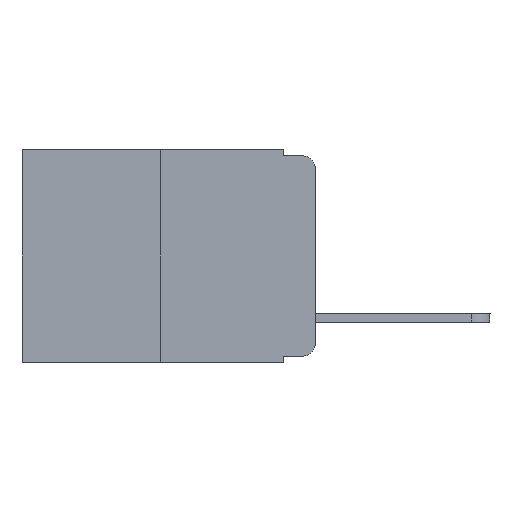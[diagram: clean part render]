
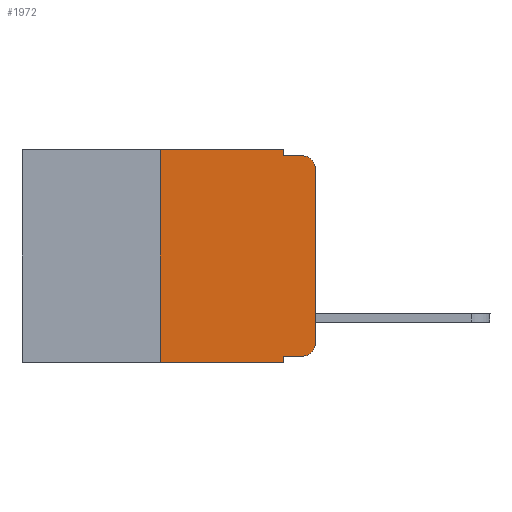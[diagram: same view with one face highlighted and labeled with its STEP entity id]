
A CAD part, left-side view. The second image highlights one B-rep face of the part: STEP entity #1972.
In plain terms, the highlighted planar face has unit normal (-1, 0, 0).
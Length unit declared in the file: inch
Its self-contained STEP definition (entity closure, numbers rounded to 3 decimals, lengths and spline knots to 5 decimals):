
#208 = DIRECTION ( 'NONE',  ( 0., 0., 1. ) ) ;
#659 = LINE ( 'NONE', #13359, #13263 ) ;
#694 = CARTESIAN_POINT ( 'NONE',  ( 0., 0.473, 0. ) ) ;
#1264 = DIRECTION ( 'NONE',  ( 0., 0., -1. ) ) ;
#1490 = CARTESIAN_POINT ( 'NONE',  ( 0., 0.051, -0.333 ) ) ;
#1658 = DIRECTION ( 'NONE',  ( 0., -1., 0. ) ) ;
#1783 = CARTESIAN_POINT ( 'NONE',  ( 0., 0.25, -0.343 ) ) ;
#1972 = ADVANCED_FACE ( 'NONE', ( #10226 ), #14744, .F. ) ;
#3472 = VERTEX_POINT ( 'NONE', #1783 ) ;
#3573 = ORIENTED_EDGE ( 'NONE', *, *, #5181, .T. ) ;
#3999 = CARTESIAN_POINT ( 'NONE',  ( 0., 0.051, -0.333 ) ) ;
#4110 = DIRECTION ( 'NONE',  ( -1., 0., 0. ) ) ;
#4302 = ORIENTED_EDGE ( 'NONE', *, *, #16141, .F. ) ;
#4472 = ORIENTED_EDGE ( 'NONE', *, *, #11755, .F. ) ;
#5054 = VERTEX_POINT ( 'NONE', #16000 ) ;
#5181 = EDGE_CURVE ( 'NONE', #12700, #6985, #9974, .T. ) ;
#5601 = DIRECTION ( 'NONE',  ( 0., 0., -1. ) ) ;
#5642 = EDGE_CURVE ( 'NONE', #3472, #6374, #10042, .T. ) ;
#5672 = CIRCLE ( 'NONE', #19744, 0.02 ) ;
#5918 = VECTOR ( 'NONE', #6756, 39.37008 ) ;
#6089 = CARTESIAN_POINT ( 'NONE',  ( 0., 0.25, 0. ) ) ;
#6374 = VERTEX_POINT ( 'NONE', #12897 ) ;
#6541 = CARTESIAN_POINT ( 'NONE',  ( 0., 0., -0.313 ) ) ;
#6551 = VECTOR ( 'NONE', #19819, 39.37008 ) ;
#6756 = DIRECTION ( 'NONE',  ( 0., -1., 0. ) ) ;
#6985 = VERTEX_POINT ( 'NONE', #12706 ) ;
#7317 = ORIENTED_EDGE ( 'NONE', *, *, #8917, .T. ) ;
#7386 = LINE ( 'NONE', #13646, #15836 ) ;
#7687 = VERTEX_POINT ( 'NONE', #7826 ) ;
#7826 = CARTESIAN_POINT ( 'NONE',  ( 0., 0.051, 0. ) ) ;
#8435 = DIRECTION ( 'NONE',  ( 0., 0., -1. ) ) ;
#8522 = ORIENTED_EDGE ( 'NONE', *, *, #5642, .T. ) ;
#8561 = DIRECTION ( 'NONE',  ( -1., 0., 0. ) ) ;
#8579 = CARTESIAN_POINT ( 'NONE',  ( 0., 0.473, -0.343 ) ) ;
#8917 = EDGE_CURVE ( 'NONE', #20241, #9786, #17738, .T. ) ;
#9378 = CARTESIAN_POINT ( 'NONE',  ( 0., 0.051, -0.01 ) ) ;
#9562 = CARTESIAN_POINT ( 'NONE',  ( 0., 0.473, 0. ) ) ;
#9786 = VERTEX_POINT ( 'NONE', #18335 ) ;
#9863 = DIRECTION ( 'NONE',  ( 0., -1., 0. ) ) ;
#9974 = LINE ( 'NONE', #3999, #16720 ) ;
#10042 = LINE ( 'NONE', #8579, #5918 ) ;
#10110 = CARTESIAN_POINT ( 'NONE',  ( 0., 0.02, -0.03 ) ) ;
#10226 = FACE_OUTER_BOUND ( 'NONE', #14265, .T. ) ;
#10424 = CARTESIAN_POINT ( 'NONE',  ( 0., 0., -0.03 ) ) ;
#11413 = CARTESIAN_POINT ( 'NONE',  ( 0., 0.051, -0.01 ) ) ;
#11673 = VERTEX_POINT ( 'NONE', #9378 ) ;
#11755 = EDGE_CURVE ( 'NONE', #12700, #6374, #659, .T. ) ;
#12264 = ORIENTED_EDGE ( 'NONE', *, *, #19534, .T. ) ;
#12394 = VECTOR ( 'NONE', #1658, 39.37008 ) ;
#12700 = VERTEX_POINT ( 'NONE', #1490 ) ;
#12706 = CARTESIAN_POINT ( 'NONE',  ( 0., 0.02, -0.333 ) ) ;
#12897 = CARTESIAN_POINT ( 'NONE',  ( 0., 0.051, -0.343 ) ) ;
#13050 = LINE ( 'NONE', #11413, #14045 ) ;
#13263 = VECTOR ( 'NONE', #8435, 39.37008 ) ;
#13359 = CARTESIAN_POINT ( 'NONE',  ( 0., 0.051, 0. ) ) ;
#13646 = CARTESIAN_POINT ( 'NONE',  ( 0., 0., 0. ) ) ;
#13983 = LINE ( 'NONE', #18255, #14373 ) ;
#14045 = VECTOR ( 'NONE', #16410, 39.37008 ) ;
#14265 = EDGE_LOOP ( 'NONE', ( #12264, #7317, #20155, #17011, #14836, #4302, #8522, #4472, #3573, #19899 ) ) ;
#14373 = VECTOR ( 'NONE', #1264, 39.37008 ) ;
#14385 = LINE ( 'NONE', #9562, #12394 ) ;
#14744 = PLANE ( 'NONE',  #20059 ) ;
#14786 = EDGE_CURVE ( 'NONE', #7687, #11673, #13983, .T. ) ;
#14836 = ORIENTED_EDGE ( 'NONE', *, *, #14855, .F. ) ;
#14839 = DIRECTION ( 'NONE',  ( 0., 0., -1. ) ) ;
#14855 = EDGE_CURVE ( 'NONE', #5054, #7687, #14385, .T. ) ;
#15091 = EDGE_CURVE ( 'NONE', #11673, #9786, #13050, .T. ) ;
#15764 = AXIS2_PLACEMENT_3D ( 'NONE', #10110, #8561, #14839 ) ;
#15836 = VECTOR ( 'NONE', #208, 39.37008 ) ;
#16000 = CARTESIAN_POINT ( 'NONE',  ( 0., 0.25, 0. ) ) ;
#16141 = EDGE_CURVE ( 'NONE', #3472, #5054, #18670, .T. ) ;
#16410 = DIRECTION ( 'NONE',  ( 0., -1., 0. ) ) ;
#16568 = DIRECTION ( 'NONE',  ( 1., 0., 0. ) ) ;
#16720 = VECTOR ( 'NONE', #9863, 39.37008 ) ;
#17011 = ORIENTED_EDGE ( 'NONE', *, *, #14786, .F. ) ;
#17036 = VERTEX_POINT ( 'NONE', #6541 ) ;
#17738 = CIRCLE ( 'NONE', #15764, 0.02 ) ;
#18139 = CARTESIAN_POINT ( 'NONE',  ( 0., 0.02, -0.313 ) ) ;
#18255 = CARTESIAN_POINT ( 'NONE',  ( 0., 0.051, 0. ) ) ;
#18335 = CARTESIAN_POINT ( 'NONE',  ( 0., 0.02, -0.01 ) ) ;
#18448 = DIRECTION ( 'NONE',  ( 0., 0., -1. ) ) ;
#18670 = LINE ( 'NONE', #6089, #6551 ) ;
#19406 = EDGE_CURVE ( 'NONE', #6985, #17036, #5672, .T. ) ;
#19534 = EDGE_CURVE ( 'NONE', #17036, #20241, #7386, .T. ) ;
#19744 = AXIS2_PLACEMENT_3D ( 'NONE', #18139, #4110, #18448 ) ;
#19819 = DIRECTION ( 'NONE',  ( 0., 0., 1. ) ) ;
#19899 = ORIENTED_EDGE ( 'NONE', *, *, #19406, .T. ) ;
#20059 = AXIS2_PLACEMENT_3D ( 'NONE', #694, #16568, #5601 ) ;
#20155 = ORIENTED_EDGE ( 'NONE', *, *, #15091, .F. ) ;
#20241 = VERTEX_POINT ( 'NONE', #10424 ) ;
